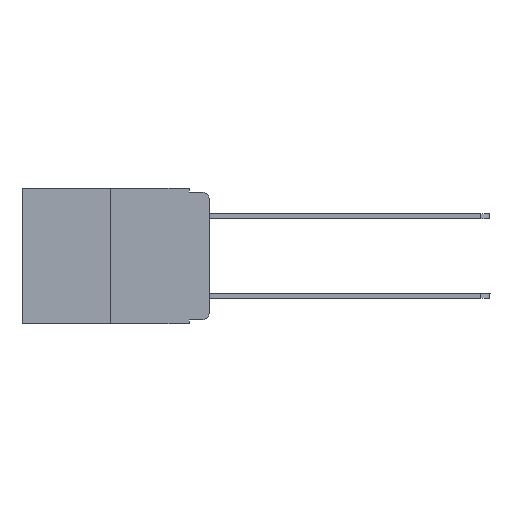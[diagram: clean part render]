
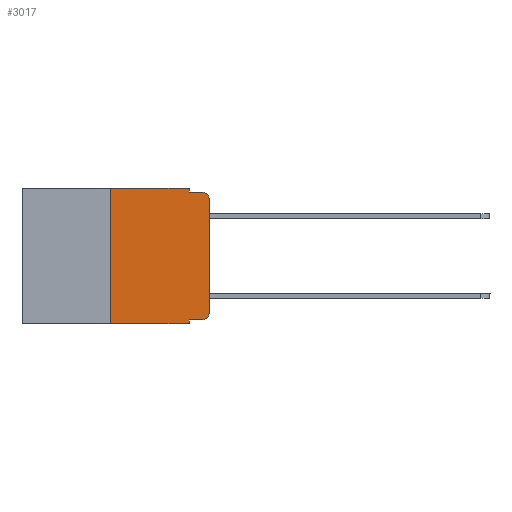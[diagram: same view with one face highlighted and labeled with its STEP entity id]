
A CAD part, left-side view. The second image highlights one B-rep face of the part: STEP entity #3017.
In plain terms, the highlighted planar face has unit normal (-1, 0, 0).
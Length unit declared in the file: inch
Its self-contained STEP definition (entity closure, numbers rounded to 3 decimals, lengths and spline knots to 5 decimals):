
#22 = DIRECTION ( 'NONE',  ( 0., -1., 0. ) ) ;
#189 = EDGE_CURVE ( 'NONE', #5155, #7633, #2938, .T. ) ;
#232 = EDGE_CURVE ( 'NONE', #5548, #4901, #11478, .T. ) ;
#255 = DIRECTION ( 'NONE',  ( 1., 0., 0. ) ) ;
#298 = CARTESIAN_POINT ( 'NONE',  ( 0., 0., 0. ) ) ;
#370 = VECTOR ( 'NONE', #14001, 39.37008 ) ;
#385 = AXIS2_PLACEMENT_3D ( 'NONE', #8476, #255, #1689 ) ;
#483 = EDGE_CURVE ( 'NONE', #5680, #14694, #8384, .T. ) ;
#489 = FACE_OUTER_BOUND ( 'NONE', #11836, .T. ) ;
#532 = EDGE_CURVE ( 'NONE', #11604, #7633, #13261, .T. ) ;
#673 = EDGE_CURVE ( 'NONE', #10087, #10217, #10381, .T. ) ;
#717 = CARTESIAN_POINT ( 'NONE',  ( 0., 0.02, -0.03 ) ) ;
#722 = ORIENTED_EDGE ( 'NONE', *, *, #11412, .F. ) ;
#847 = CARTESIAN_POINT ( 'NONE',  ( 0., 0.051, -0.01 ) ) ;
#960 = EDGE_CURVE ( 'NONE', #10217, #5155, #11750, .T. ) ;
#983 = LINE ( 'NONE', #5513, #3954 ) ;
#984 = VECTOR ( 'NONE', #7492, 39.37008 ) ;
#1193 = LINE ( 'NONE', #1261, #9964 ) ;
#1261 = CARTESIAN_POINT ( 'NONE',  ( 0., 0.051, 0. ) ) ;
#1266 = EDGE_CURVE ( 'NONE', #5548, #5680, #983, .T. ) ;
#1461 = VECTOR ( 'NONE', #6564, 39.37008 ) ;
#1484 = ORIENTED_EDGE ( 'NONE', *, *, #483, .F. ) ;
#1689 = DIRECTION ( 'NONE',  ( 0., 0., -1. ) ) ;
#1963 = CARTESIAN_POINT ( 'NONE',  ( 0., 0.02, -0.313 ) ) ;
#2057 = DIRECTION ( 'NONE',  ( -1., 0., 0. ) ) ;
#2746 = AXIS2_PLACEMENT_3D ( 'NONE', #1963, #6496, #14661 ) ;
#2938 = CIRCLE ( 'NONE', #10583, 0.02 ) ;
#3017 = ADVANCED_FACE ( 'NONE', ( #489 ), #3917, .F. ) ;
#3026 = ORIENTED_EDGE ( 'NONE', *, *, #189, .T. ) ;
#3723 = ORIENTED_EDGE ( 'NONE', *, *, #1266, .F. ) ;
#3917 = PLANE ( 'NONE',  #385 ) ;
#3954 = VECTOR ( 'NONE', #6109, 39.37008 ) ;
#4251 = CARTESIAN_POINT ( 'NONE',  ( 0., 0.02, -0.333 ) ) ;
#4891 = CARTESIAN_POINT ( 'NONE',  ( 0., 0.02, -0.01 ) ) ;
#4901 = VERTEX_POINT ( 'NONE', #13411 ) ;
#4965 = VERTEX_POINT ( 'NONE', #11246 ) ;
#5003 = CARTESIAN_POINT ( 'NONE',  ( 0., 0.051, 0. ) ) ;
#5037 = ORIENTED_EDGE ( 'NONE', *, *, #5981, .F. ) ;
#5155 = VERTEX_POINT ( 'NONE', #10559 ) ;
#5513 = CARTESIAN_POINT ( 'NONE',  ( 0., 0.25, 0. ) ) ;
#5526 = ORIENTED_EDGE ( 'NONE', *, *, #532, .F. ) ;
#5548 = VERTEX_POINT ( 'NONE', #9179 ) ;
#5680 = VERTEX_POINT ( 'NONE', #10544 ) ;
#5981 = EDGE_CURVE ( 'NONE', #4965, #4901, #1193, .T. ) ;
#6109 = DIRECTION ( 'NONE',  ( 0., 0., 1. ) ) ;
#6496 = DIRECTION ( 'NONE',  ( -1., 0., 0. ) ) ;
#6564 = DIRECTION ( 'NONE',  ( 0., -1., 0. ) ) ;
#7492 = DIRECTION ( 'NONE',  ( 0., 0., -1. ) ) ;
#7536 = ORIENTED_EDGE ( 'NONE', *, *, #673, .T. ) ;
#7633 = VERTEX_POINT ( 'NONE', #4891 ) ;
#7810 = ORIENTED_EDGE ( 'NONE', *, *, #232, .T. ) ;
#8384 = LINE ( 'NONE', #10571, #13024 ) ;
#8476 = CARTESIAN_POINT ( 'NONE',  ( 0., 0.473, 0. ) ) ;
#8658 = VECTOR ( 'NONE', #22, 39.37008 ) ;
#8813 = DIRECTION ( 'NONE',  ( 0., -1., 0. ) ) ;
#8833 = DIRECTION ( 'NONE',  ( 0., 0., -1. ) ) ;
#9045 = CARTESIAN_POINT ( 'NONE',  ( 0., 0., -0.313 ) ) ;
#9179 = CARTESIAN_POINT ( 'NONE',  ( 0., 0.25, -0.343 ) ) ;
#9964 = VECTOR ( 'NONE', #14636, 39.37008 ) ;
#10020 = EDGE_CURVE ( 'NONE', #4965, #10087, #10936, .T. ) ;
#10087 = VERTEX_POINT ( 'NONE', #4251 ) ;
#10154 = ORIENTED_EDGE ( 'NONE', *, *, #960, .T. ) ;
#10217 = VERTEX_POINT ( 'NONE', #9045 ) ;
#10229 = ORIENTED_EDGE ( 'NONE', *, *, #10020, .T. ) ;
#10348 = CARTESIAN_POINT ( 'NONE',  ( 0., 0.051, -0.01 ) ) ;
#10381 = CIRCLE ( 'NONE', #2746, 0.02 ) ;
#10544 = CARTESIAN_POINT ( 'NONE',  ( 0., 0.25, 0. ) ) ;
#10559 = CARTESIAN_POINT ( 'NONE',  ( 0., 0., -0.03 ) ) ;
#10571 = CARTESIAN_POINT ( 'NONE',  ( 0., 0.473, 0. ) ) ;
#10583 = AXIS2_PLACEMENT_3D ( 'NONE', #717, #2057, #8833 ) ;
#10936 = LINE ( 'NONE', #12207, #1461 ) ;
#11246 = CARTESIAN_POINT ( 'NONE',  ( 0., 0.051, -0.333 ) ) ;
#11412 = EDGE_CURVE ( 'NONE', #14694, #11604, #13282, .T. ) ;
#11478 = LINE ( 'NONE', #12459, #8658 ) ;
#11604 = VERTEX_POINT ( 'NONE', #10348 ) ;
#11750 = LINE ( 'NONE', #298, #370 ) ;
#11836 = EDGE_LOOP ( 'NONE', ( #10154, #3026, #5526, #722, #1484, #3723, #7810, #5037, #10229, #7536 ) ) ;
#12207 = CARTESIAN_POINT ( 'NONE',  ( 0., 0.051, -0.333 ) ) ;
#12319 = CARTESIAN_POINT ( 'NONE',  ( 0., 0.051, 0. ) ) ;
#12459 = CARTESIAN_POINT ( 'NONE',  ( 0., 0.473, -0.343 ) ) ;
#13024 = VECTOR ( 'NONE', #14161, 39.37008 ) ;
#13261 = LINE ( 'NONE', #847, #13741 ) ;
#13282 = LINE ( 'NONE', #12319, #984 ) ;
#13411 = CARTESIAN_POINT ( 'NONE',  ( 0., 0.051, -0.343 ) ) ;
#13741 = VECTOR ( 'NONE', #8813, 39.37008 ) ;
#14001 = DIRECTION ( 'NONE',  ( 0., 0., 1. ) ) ;
#14161 = DIRECTION ( 'NONE',  ( 0., -1., 0. ) ) ;
#14636 = DIRECTION ( 'NONE',  ( 0., 0., -1. ) ) ;
#14661 = DIRECTION ( 'NONE',  ( 0., 0., -1. ) ) ;
#14694 = VERTEX_POINT ( 'NONE', #5003 ) ;
